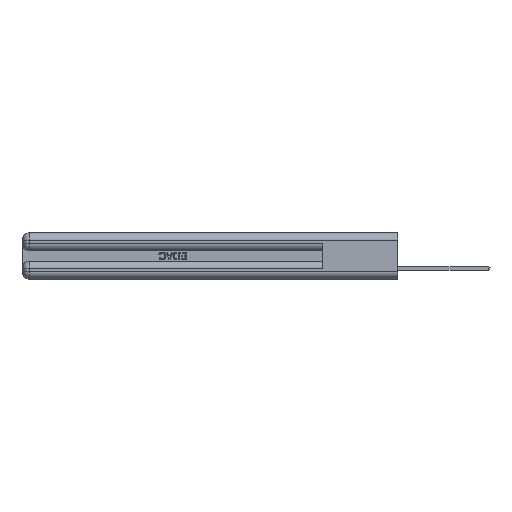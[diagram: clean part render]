
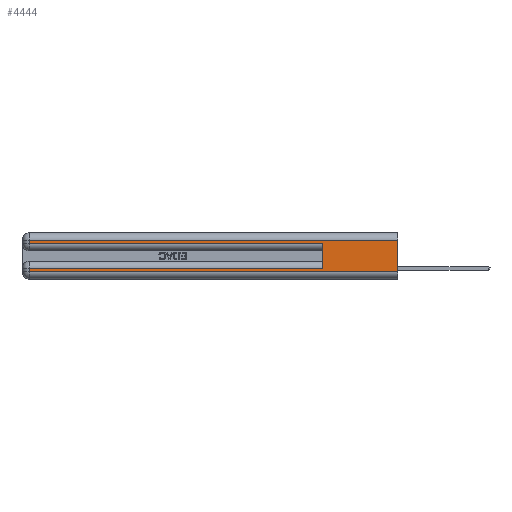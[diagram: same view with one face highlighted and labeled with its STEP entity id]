
A CAD part, left-side view. The second image highlights one B-rep face of the part: STEP entity #4444.
In plain terms, the highlighted planar face has unit normal (-1, 0, 0).
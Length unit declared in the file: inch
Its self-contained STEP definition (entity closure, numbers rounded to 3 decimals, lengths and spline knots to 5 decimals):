
#159 = ORIENTED_EDGE ( 'NONE', *, *, #46110, .T. ) ;
#1687 = DIRECTION ( 'NONE',  ( 0., 0., -1. ) ) ;
#1839 = EDGE_CURVE ( 'NONE', #33013, #12977, #24233, .T. ) ;
#2369 = EDGE_CURVE ( 'NONE', #7382, #17544, #40391, .T. ) ;
#4192 = ORIENTED_EDGE ( 'NONE', *, *, #42349, .T. ) ;
#4444 = ADVANCED_FACE ( 'NONE', ( #28970 ), #11287, .F. ) ;
#4467 = VERTEX_POINT ( 'NONE', #50040 ) ;
#4979 = VECTOR ( 'NONE', #51533, 39.37008 ) ;
#7382 = VERTEX_POINT ( 'NONE', #50384 ) ;
#8681 = LINE ( 'NONE', #34835, #41703 ) ;
#10258 = ORIENTED_EDGE ( 'NONE', *, *, #2369, .T. ) ;
#10949 = AXIS2_PLACEMENT_3D ( 'NONE', #27464, #30764, #36076 ) ;
#10996 = DIRECTION ( 'NONE',  ( 0., 1., 0. ) ) ;
#11287 = PLANE ( 'NONE',  #10949 ) ;
#11980 = CARTESIAN_POINT ( 'NONE',  ( 0., 0., 0.06 ) ) ;
#12119 = CARTESIAN_POINT ( 'NONE',  ( 0., 2.94, 0.06 ) ) ;
#12560 = CARTESIAN_POINT ( 'NONE',  ( 0., 0., 0.37 ) ) ;
#12977 = VERTEX_POINT ( 'NONE', #11980 ) ;
#13052 = DIRECTION ( 'NONE',  ( 0., -1., 0. ) ) ;
#14041 = CARTESIAN_POINT ( 'NONE',  ( 0., 2.94, 0.37 ) ) ;
#14975 = VERTEX_POINT ( 'NONE', #16705 ) ;
#15483 = EDGE_CURVE ( 'NONE', #7382, #14975, #43639, .T. ) ;
#16073 = EDGE_CURVE ( 'NONE', #33013, #4467, #8681, .T. ) ;
#16295 = LINE ( 'NONE', #40526, #17520 ) ;
#16705 = CARTESIAN_POINT ( 'NONE',  ( 0., 0.6, 0.285 ) ) ;
#17028 = CARTESIAN_POINT ( 'NONE',  ( 0., 2.94, 0.285 ) ) ;
#17520 = VECTOR ( 'NONE', #44217, 39.37008 ) ;
#17544 = VERTEX_POINT ( 'NONE', #24348 ) ;
#19118 = VECTOR ( 'NONE', #13052, 39.37008 ) ;
#24077 = LINE ( 'NONE', #29406, #19118 ) ;
#24233 = LINE ( 'NONE', #12560, #44219 ) ;
#24348 = CARTESIAN_POINT ( 'NONE',  ( 0., 2.94, 0.085 ) ) ;
#27464 = CARTESIAN_POINT ( 'NONE',  ( 0., 0., 0.37 ) ) ;
#28970 = FACE_OUTER_BOUND ( 'NONE', #41307, .T. ) ;
#29332 = ORIENTED_EDGE ( 'NONE', *, *, #16073, .T. ) ;
#29406 = CARTESIAN_POINT ( 'NONE',  ( 0., 0., 0.06 ) ) ;
#30139 = ORIENTED_EDGE ( 'NONE', *, *, #32275, .T. ) ;
#30717 = VERTEX_POINT ( 'NONE', #17028 ) ;
#30764 = DIRECTION ( 'NONE',  ( 1., 0., 0. ) ) ;
#30936 = CARTESIAN_POINT ( 'NONE',  ( 0., 2.94, 0.37 ) ) ;
#31883 = DIRECTION ( 'NONE',  ( 0., 0., -1. ) ) ;
#32247 = CARTESIAN_POINT ( 'NONE',  ( 0., 0., 0.085 ) ) ;
#32275 = EDGE_CURVE ( 'NONE', #30717, #14975, #16295, .T. ) ;
#33013 = VERTEX_POINT ( 'NONE', #47847 ) ;
#34337 = VECTOR ( 'NONE', #47039, 39.37008 ) ;
#34835 = CARTESIAN_POINT ( 'NONE',  ( 0., 0., 0.31 ) ) ;
#35511 = VERTEX_POINT ( 'NONE', #12119 ) ;
#36076 = DIRECTION ( 'NONE',  ( 0., 0., -1. ) ) ;
#37606 = EDGE_CURVE ( 'NONE', #17544, #35511, #49499, .T. ) ;
#38653 = ORIENTED_EDGE ( 'NONE', *, *, #37606, .T. ) ;
#39961 = DIRECTION ( 'NONE',  ( 0., 1., 0. ) ) ;
#40391 = LINE ( 'NONE', #32247, #42946 ) ;
#40526 = CARTESIAN_POINT ( 'NONE',  ( 0., 0., 0.285 ) ) ;
#41307 = EDGE_LOOP ( 'NONE', ( #45030, #29332, #159, #30139, #42194, #10258, #38653, #4192 ) ) ;
#41703 = VECTOR ( 'NONE', #10996, 39.37008 ) ;
#41933 = CARTESIAN_POINT ( 'NONE',  ( 0., 0.6, 0.145 ) ) ;
#42194 = ORIENTED_EDGE ( 'NONE', *, *, #15483, .F. ) ;
#42349 = EDGE_CURVE ( 'NONE', #35511, #12977, #24077, .T. ) ;
#42946 = VECTOR ( 'NONE', #39961, 39.37008 ) ;
#43283 = VECTOR ( 'NONE', #1687, 39.37008 ) ;
#43639 = LINE ( 'NONE', #41933, #4979 ) ;
#44217 = DIRECTION ( 'NONE',  ( 0., -1., 0. ) ) ;
#44219 = VECTOR ( 'NONE', #31883, 39.37008 ) ;
#45030 = ORIENTED_EDGE ( 'NONE', *, *, #1839, .F. ) ;
#46110 = EDGE_CURVE ( 'NONE', #4467, #30717, #46224, .T. ) ;
#46224 = LINE ( 'NONE', #30936, #34337 ) ;
#47039 = DIRECTION ( 'NONE',  ( 0., 0., -1. ) ) ;
#47847 = CARTESIAN_POINT ( 'NONE',  ( 0., 0., 0.31 ) ) ;
#49499 = LINE ( 'NONE', #14041, #43283 ) ;
#50040 = CARTESIAN_POINT ( 'NONE',  ( 0., 2.94, 0.31 ) ) ;
#50384 = CARTESIAN_POINT ( 'NONE',  ( 0., 0.6, 0.085 ) ) ;
#51533 = DIRECTION ( 'NONE',  ( 0., 0., 1. ) ) ;
